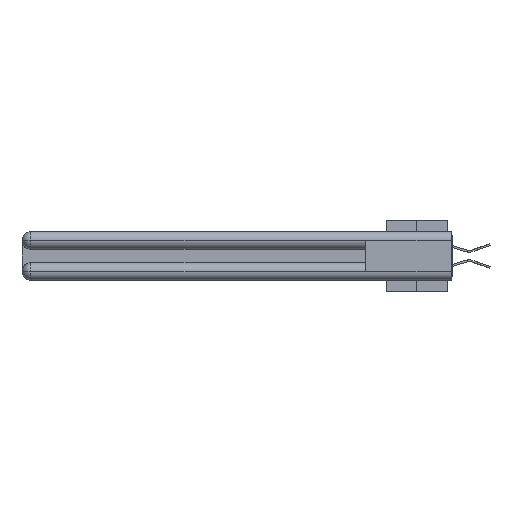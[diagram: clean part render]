
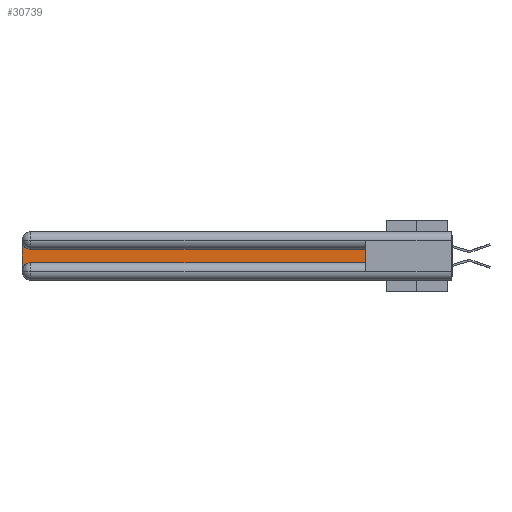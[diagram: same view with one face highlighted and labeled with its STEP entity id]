
A CAD part, left-side view. The second image highlights one B-rep face of the part: STEP entity #30739.
In plain terms, the highlighted planar face has unit normal (-1, 0, 0).
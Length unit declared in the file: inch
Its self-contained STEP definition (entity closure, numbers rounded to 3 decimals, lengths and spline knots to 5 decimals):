
#417 = DIRECTION ( 'NONE',  ( 1., 0., 0. ) ) ;
#1103 = VERTEX_POINT ( 'NONE', #16317 ) ;
#1957 = AXIS2_PLACEMENT_3D ( 'NONE', #22331, #24354, #27818 ) ;
#2128 = EDGE_CURVE ( 'NONE', #11132, #16831, #11686, .T. ) ;
#2695 = VERTEX_POINT ( 'NONE', #16861 ) ;
#4191 = ORIENTED_EDGE ( 'NONE', *, *, #27969, .T. ) ;
#4448 = CARTESIAN_POINT ( 'NONE',  ( 0.075, 3., -0.2175 ) ) ;
#5291 = DIRECTION ( 'NONE',  ( 1., 0., 0. ) ) ;
#5333 = VECTOR ( 'NONE', #6780, 39.37008 ) ;
#5820 = VECTOR ( 'NONE', #37252, 39.37008 ) ;
#6190 = LINE ( 'NONE', #4448, #22506 ) ;
#6780 = DIRECTION ( 'NONE',  ( 0., 1., 0. ) ) ;
#7491 = VERTEX_POINT ( 'NONE', #37929 ) ;
#8085 = CARTESIAN_POINT ( 'NONE',  ( 0.075, 2.94, -0.2175 ) ) ;
#8230 = EDGE_CURVE ( 'NONE', #16831, #7491, #36039, .T. ) ;
#8507 = ORIENTED_EDGE ( 'NONE', *, *, #14137, .T. ) ;
#10264 = CARTESIAN_POINT ( 'NONE',  ( 0.075, 0.6, -0.1225 ) ) ;
#11132 = VERTEX_POINT ( 'NONE', #18257 ) ;
#11359 = ORIENTED_EDGE ( 'NONE', *, *, #23218, .T. ) ;
#11686 = CIRCLE ( 'NONE', #40720, 0.06 ) ;
#13198 = DIRECTION ( 'NONE',  ( 0., 0., -1. ) ) ;
#14137 = EDGE_CURVE ( 'NONE', #1103, #11132, #6190, .T. ) ;
#14263 = PLANE ( 'NONE',  #18211 ) ;
#14677 = CARTESIAN_POINT ( 'NONE',  ( 0.075, 0.6, -0.2175 ) ) ;
#16317 = CARTESIAN_POINT ( 'NONE',  ( 0.075, 3., -0.0625 ) ) ;
#16831 = VERTEX_POINT ( 'NONE', #8085 ) ;
#16861 = CARTESIAN_POINT ( 'NONE',  ( 0.075, 0.6, -0.1225 ) ) ;
#16907 = ORIENTED_EDGE ( 'NONE', *, *, #2128, .T. ) ;
#18126 = CARTESIAN_POINT ( 'NONE',  ( 0.075, 0.6, -0.2175 ) ) ;
#18211 = AXIS2_PLACEMENT_3D ( 'NONE', #36849, #5291, #27402 ) ;
#18257 = CARTESIAN_POINT ( 'NONE',  ( 0.075, 3., -0.2775 ) ) ;
#19275 = VERTEX_POINT ( 'NONE', #36517 ) ;
#22331 = CARTESIAN_POINT ( 'NONE',  ( 0.075, 2.94, -0.0625 ) ) ;
#22506 = VECTOR ( 'NONE', #33089, 39.37008 ) ;
#23218 = EDGE_CURVE ( 'NONE', #2695, #19275, #37539, .T. ) ;
#24354 = DIRECTION ( 'NONE',  ( 1., 0., 0. ) ) ;
#25330 = VECTOR ( 'NONE', #36714, 39.37008 ) ;
#26803 = EDGE_LOOP ( 'NONE', ( #11359, #4191, #8507, #16907, #32330, #40194 ) ) ;
#27402 = DIRECTION ( 'NONE',  ( 0., 0., -1. ) ) ;
#27818 = DIRECTION ( 'NONE',  ( 0., 0., -1. ) ) ;
#27969 = EDGE_CURVE ( 'NONE', #19275, #1103, #40134, .T. ) ;
#28265 = CARTESIAN_POINT ( 'NONE',  ( 0.075, 2.94, -0.2775 ) ) ;
#30739 = ADVANCED_FACE ( 'NONE', ( #34322 ), #14263, .F. ) ;
#31458 = EDGE_CURVE ( 'NONE', #7491, #2695, #37745, .T. ) ;
#32330 = ORIENTED_EDGE ( 'NONE', *, *, #8230, .T. ) ;
#33089 = DIRECTION ( 'NONE',  ( 0., 0., -1. ) ) ;
#34322 = FACE_OUTER_BOUND ( 'NONE', #26803, .T. ) ;
#36039 = LINE ( 'NONE', #18126, #5820 ) ;
#36517 = CARTESIAN_POINT ( 'NONE',  ( 0.075, 2.94, -0.1225 ) ) ;
#36714 = DIRECTION ( 'NONE',  ( 0., 0., 1. ) ) ;
#36849 = CARTESIAN_POINT ( 'NONE',  ( 0.075, 3., -0.1225 ) ) ;
#37252 = DIRECTION ( 'NONE',  ( 0., -1., 0. ) ) ;
#37539 = LINE ( 'NONE', #10264, #5333 ) ;
#37745 = LINE ( 'NONE', #14677, #25330 ) ;
#37929 = CARTESIAN_POINT ( 'NONE',  ( 0.075, 0.6, -0.2175 ) ) ;
#40134 = CIRCLE ( 'NONE', #1957, 0.06 ) ;
#40194 = ORIENTED_EDGE ( 'NONE', *, *, #31458, .T. ) ;
#40720 = AXIS2_PLACEMENT_3D ( 'NONE', #28265, #417, #13198 ) ;
